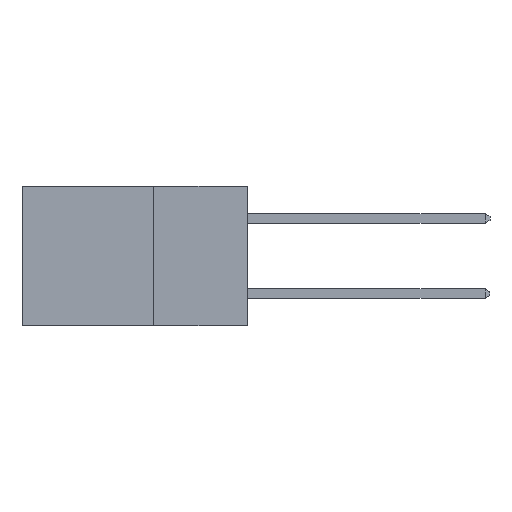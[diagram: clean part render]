
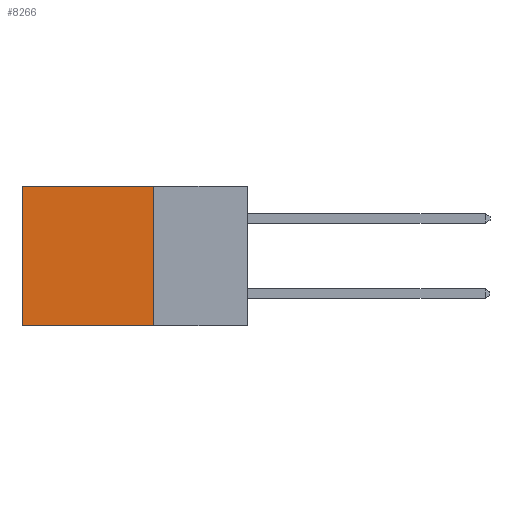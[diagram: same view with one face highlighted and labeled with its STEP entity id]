
A CAD part, left-side view. The second image highlights one B-rep face of the part: STEP entity #8266.
In plain terms, the highlighted planar face has unit normal (-1, 0, 0).
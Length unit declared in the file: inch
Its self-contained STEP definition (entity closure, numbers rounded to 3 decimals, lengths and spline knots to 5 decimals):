
#717 = EDGE_CURVE ( 'NONE', #6418, #9691, #6630, .T. ) ;
#1050 = CARTESIAN_POINT ( 'NONE',  ( 0.298, 0.6, 0. ) ) ;
#1184 = VECTOR ( 'NONE', #1186, 39.37008 ) ;
#1186 = DIRECTION ( 'NONE',  ( 0., 0., -1. ) ) ;
#2356 = CARTESIAN_POINT ( 'NONE',  ( 0.298, 0.25, -0.37 ) ) ;
#2665 = DIRECTION ( 'NONE',  ( 1., 0., 0. ) ) ;
#2768 = LINE ( 'NONE', #11326, #10419 ) ;
#2850 = CARTESIAN_POINT ( 'NONE',  ( 0.298, 0.6, -0.37 ) ) ;
#2962 = VECTOR ( 'NONE', #8170, 39.37008 ) ;
#3106 = ORIENTED_EDGE ( 'NONE', *, *, #9837, .T. ) ;
#3920 = LINE ( 'NONE', #6188, #1184 ) ;
#3989 = DIRECTION ( 'NONE',  ( 0., 0., -1. ) ) ;
#4042 = VECTOR ( 'NONE', #3989, 39.37008 ) ;
#4477 = CARTESIAN_POINT ( 'NONE',  ( 0.298, 0.25, 0. ) ) ;
#5991 = EDGE_LOOP ( 'NONE', ( #3106, #10457, #10629, #8620 ) ) ;
#6188 = CARTESIAN_POINT ( 'NONE',  ( 0.298, 0.6, 0. ) ) ;
#6418 = VERTEX_POINT ( 'NONE', #10966 ) ;
#6549 = DIRECTION ( 'NONE',  ( 0., 1., 0. ) ) ;
#6630 = LINE ( 'NONE', #4477, #4042 ) ;
#6677 = VERTEX_POINT ( 'NONE', #2850 ) ;
#7028 = EDGE_CURVE ( 'NONE', #6418, #9752, #2768, .T. ) ;
#7820 = CARTESIAN_POINT ( 'NONE',  ( 0.298, 0.25, -0.37 ) ) ;
#8099 = LINE ( 'NONE', #2356, #2962 ) ;
#8170 = DIRECTION ( 'NONE',  ( 0., 1., 0. ) ) ;
#8266 = ADVANCED_FACE ( 'NONE', ( #12222 ), #8461, .F. ) ;
#8425 = CARTESIAN_POINT ( 'NONE',  ( 0.298, 0.25, 0. ) ) ;
#8461 = PLANE ( 'NONE',  #8769 ) ;
#8620 = ORIENTED_EDGE ( 'NONE', *, *, #7028, .T. ) ;
#8769 = AXIS2_PLACEMENT_3D ( 'NONE', #8425, #2665, #9401 ) ;
#9401 = DIRECTION ( 'NONE',  ( 0., 0., -1. ) ) ;
#9691 = VERTEX_POINT ( 'NONE', #7820 ) ;
#9752 = VERTEX_POINT ( 'NONE', #1050 ) ;
#9837 = EDGE_CURVE ( 'NONE', #9752, #6677, #3920, .T. ) ;
#9922 = EDGE_CURVE ( 'NONE', #9691, #6677, #8099, .T. ) ;
#10419 = VECTOR ( 'NONE', #6549, 39.37008 ) ;
#10457 = ORIENTED_EDGE ( 'NONE', *, *, #9922, .F. ) ;
#10629 = ORIENTED_EDGE ( 'NONE', *, *, #717, .F. ) ;
#10966 = CARTESIAN_POINT ( 'NONE',  ( 0.298, 0.25, 0. ) ) ;
#11326 = CARTESIAN_POINT ( 'NONE',  ( 0.298, 0.25, 0. ) ) ;
#12222 = FACE_OUTER_BOUND ( 'NONE', #5991, .T. ) ;
